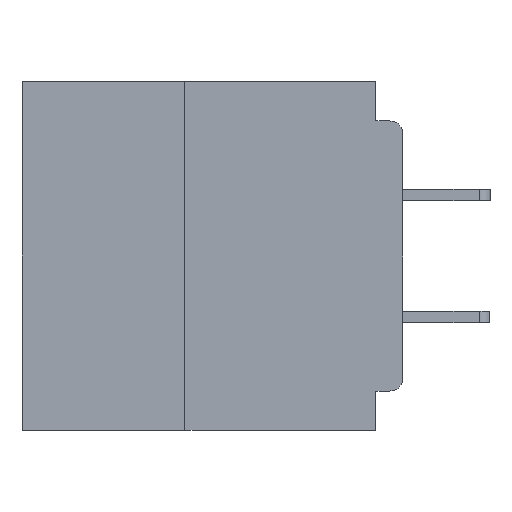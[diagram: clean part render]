
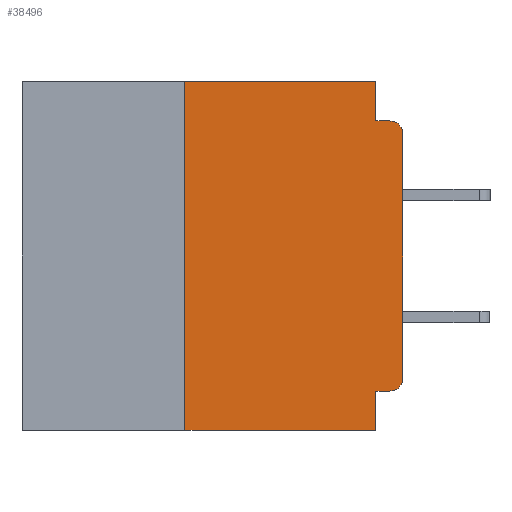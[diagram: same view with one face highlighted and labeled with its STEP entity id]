
A CAD part, left-side view. The second image highlights one B-rep face of the part: STEP entity #38496.
In plain terms, the highlighted planar face has unit normal (-1, 0, 0).
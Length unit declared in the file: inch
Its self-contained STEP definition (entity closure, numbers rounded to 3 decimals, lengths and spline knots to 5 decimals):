
#874 = ORIENTED_EDGE ( 'NONE', *, *, #28163, .F. ) ;
#1271 = VERTEX_POINT ( 'NONE', #20740 ) ;
#1314 = ORIENTED_EDGE ( 'NONE', *, *, #19221, .T. ) ;
#1406 = DIRECTION ( 'NONE',  ( 0., 0., 1. ) ) ;
#2649 = LINE ( 'NONE', #31087, #42030 ) ;
#2747 = CARTESIAN_POINT ( 'NONE',  ( 0., 0.031, -0.4 ) ) ;
#2829 = LINE ( 'NONE', #48767, #22661 ) ;
#4067 = CARTESIAN_POINT ( 'NONE',  ( 0., 0.031, 0. ) ) ;
#5427 = CARTESIAN_POINT ( 'NONE',  ( 0., 0., -0.06 ) ) ;
#6275 = FACE_OUTER_BOUND ( 'NONE', #9821, .T. ) ;
#6375 = VECTOR ( 'NONE', #11586, 39.37008 ) ;
#6575 = DIRECTION ( 'NONE',  ( -1., 0., 0. ) ) ;
#6758 = VERTEX_POINT ( 'NONE', #19259 ) ;
#6827 = DIRECTION ( 'NONE',  ( 0., 0., -1. ) ) ;
#8159 = LINE ( 'NONE', #26283, #47290 ) ;
#8283 = VERTEX_POINT ( 'NONE', #17523 ) ;
#8620 = VERTEX_POINT ( 'NONE', #50579 ) ;
#9069 = DIRECTION ( 'NONE',  ( 1., 0., 0. ) ) ;
#9821 = EDGE_LOOP ( 'NONE', ( #1314, #24499, #28496, #31579, #37113, #49266, #49614, #874, #29516, #23062 ) ) ;
#10594 = LINE ( 'NONE', #2747, #40540 ) ;
#11586 = DIRECTION ( 'NONE',  ( 0., 0., 1. ) ) ;
#12815 = CARTESIAN_POINT ( 'NONE',  ( 0., 0.015, -0.355 ) ) ;
#14176 = AXIS2_PLACEMENT_3D ( 'NONE', #19761, #47030, #23672 ) ;
#15200 = VERTEX_POINT ( 'NONE', #36410 ) ;
#15547 = DIRECTION ( 'NONE',  ( 0., 0., -1. ) ) ;
#15613 = CARTESIAN_POINT ( 'NONE',  ( 0., 0.25, 0. ) ) ;
#15725 = VERTEX_POINT ( 'NONE', #12815 ) ;
#16953 = LINE ( 'NONE', #48661, #27331 ) ;
#17313 = DIRECTION ( 'NONE',  ( 0., -1., 0. ) ) ;
#17523 = CARTESIAN_POINT ( 'NONE',  ( 0., 0.031, -0.355 ) ) ;
#19221 = EDGE_CURVE ( 'NONE', #15200, #23280, #16953, .T. ) ;
#19259 = CARTESIAN_POINT ( 'NONE',  ( 0., 0.25, -0.4 ) ) ;
#19710 = AXIS2_PLACEMENT_3D ( 'NONE', #30099, #6575, #34019 ) ;
#19713 = EDGE_CURVE ( 'NONE', #15725, #15200, #35210, .T. ) ;
#19761 = CARTESIAN_POINT ( 'NONE',  ( 0., 0.015, -0.34 ) ) ;
#20740 = CARTESIAN_POINT ( 'NONE',  ( 0., 0.031, -0.045 ) ) ;
#20834 = EDGE_CURVE ( 'NONE', #6758, #27038, #8159, .T. ) ;
#22162 = VERTEX_POINT ( 'NONE', #15613 ) ;
#22661 = VECTOR ( 'NONE', #29312, 39.37008 ) ;
#23062 = ORIENTED_EDGE ( 'NONE', *, *, #19713, .T. ) ;
#23280 = VERTEX_POINT ( 'NONE', #5427 ) ;
#23292 = CARTESIAN_POINT ( 'NONE',  ( 0., 0.031, -0.4 ) ) ;
#23672 = DIRECTION ( 'NONE',  ( 0., 0., -1. ) ) ;
#23925 = EDGE_CURVE ( 'NONE', #1271, #8620, #44097, .T. ) ;
#24499 = ORIENTED_EDGE ( 'NONE', *, *, #35931, .T. ) ;
#24847 = LINE ( 'NONE', #34969, #6375 ) ;
#25577 = CARTESIAN_POINT ( 'NONE',  ( 0., 0., -0.355 ) ) ;
#25907 = EDGE_CURVE ( 'NONE', #45979, #1271, #2649, .T. ) ;
#26283 = CARTESIAN_POINT ( 'NONE',  ( 0., 0.437, -0.4 ) ) ;
#27038 = VERTEX_POINT ( 'NONE', #23292 ) ;
#27331 = VECTOR ( 'NONE', #1406, 39.37008 ) ;
#28163 = EDGE_CURVE ( 'NONE', #8283, #27038, #10594, .T. ) ;
#28496 = ORIENTED_EDGE ( 'NONE', *, *, #23925, .F. ) ;
#29260 = AXIS2_PLACEMENT_3D ( 'NONE', #32517, #9069, #36428 ) ;
#29312 = DIRECTION ( 'NONE',  ( 0., -1., 0. ) ) ;
#29347 = DIRECTION ( 'NONE',  ( 0., 1., 0. ) ) ;
#29516 = ORIENTED_EDGE ( 'NONE', *, *, #40040, .F. ) ;
#30099 = CARTESIAN_POINT ( 'NONE',  ( 0., 0.015, -0.06 ) ) ;
#30676 = CIRCLE ( 'NONE', #19710, 0.015 ) ;
#31087 = CARTESIAN_POINT ( 'NONE',  ( 0., 0.031, 0. ) ) ;
#31579 = ORIENTED_EDGE ( 'NONE', *, *, #25907, .F. ) ;
#32489 = VECTOR ( 'NONE', #17313, 39.37008 ) ;
#32517 = CARTESIAN_POINT ( 'NONE',  ( 0., 0.437, 0. ) ) ;
#34019 = DIRECTION ( 'NONE',  ( 0., 0., -1. ) ) ;
#34969 = CARTESIAN_POINT ( 'NONE',  ( 0., 0.25, -0.4 ) ) ;
#35210 = CIRCLE ( 'NONE', #14176, 0.015 ) ;
#35931 = EDGE_CURVE ( 'NONE', #23280, #8620, #30676, .T. ) ;
#36410 = CARTESIAN_POINT ( 'NONE',  ( 0., 0., -0.34 ) ) ;
#36428 = DIRECTION ( 'NONE',  ( 0., 0., -1. ) ) ;
#36766 = CARTESIAN_POINT ( 'NONE',  ( 0., 0., -0.045 ) ) ;
#37113 = ORIENTED_EDGE ( 'NONE', *, *, #50134, .F. ) ;
#37460 = LINE ( 'NONE', #25577, #47868 ) ;
#37680 = EDGE_CURVE ( 'NONE', #6758, #22162, #24847, .T. ) ;
#38496 = ADVANCED_FACE ( 'NONE', ( #6275 ), #44121, .F. ) ;
#40040 = EDGE_CURVE ( 'NONE', #15725, #8283, #37460, .T. ) ;
#40540 = VECTOR ( 'NONE', #6827, 39.37008 ) ;
#41824 = DIRECTION ( 'NONE',  ( 0., -1., 0. ) ) ;
#42030 = VECTOR ( 'NONE', #15547, 39.37008 ) ;
#44097 = LINE ( 'NONE', #36766, #32489 ) ;
#44121 = PLANE ( 'NONE',  #29260 ) ;
#45979 = VERTEX_POINT ( 'NONE', #4067 ) ;
#47030 = DIRECTION ( 'NONE',  ( -1., 0., 0. ) ) ;
#47290 = VECTOR ( 'NONE', #41824, 39.37008 ) ;
#47868 = VECTOR ( 'NONE', #29347, 39.37008 ) ;
#48661 = CARTESIAN_POINT ( 'NONE',  ( 0., 0., 0. ) ) ;
#48767 = CARTESIAN_POINT ( 'NONE',  ( 0., 0.437, 0. ) ) ;
#49266 = ORIENTED_EDGE ( 'NONE', *, *, #37680, .F. ) ;
#49614 = ORIENTED_EDGE ( 'NONE', *, *, #20834, .T. ) ;
#50134 = EDGE_CURVE ( 'NONE', #22162, #45979, #2829, .T. ) ;
#50579 = CARTESIAN_POINT ( 'NONE',  ( 0., 0.015, -0.045 ) ) ;
